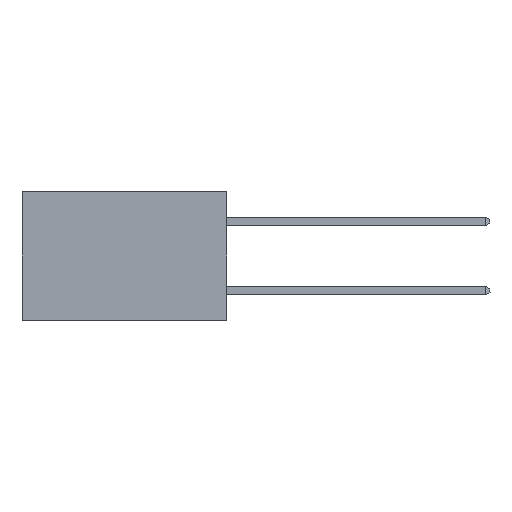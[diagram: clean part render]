
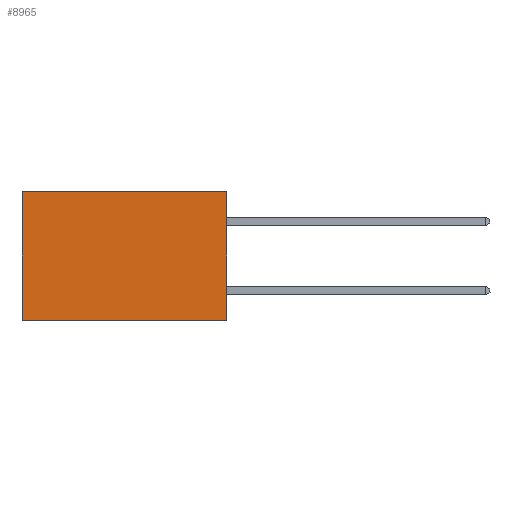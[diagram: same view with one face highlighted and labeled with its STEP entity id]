
A CAD part, left-side view. The second image highlights one B-rep face of the part: STEP entity #8965.
In plain terms, the highlighted planar face has unit normal (-1, 0, 0).
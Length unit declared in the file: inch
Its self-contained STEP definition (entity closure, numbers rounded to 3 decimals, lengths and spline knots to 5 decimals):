
#367 = CARTESIAN_POINT ( 'NONE',  ( 0.277, 0., 0. ) ) ;
#371 = VERTEX_POINT ( 'NONE', #10966 ) ;
#511 = VECTOR ( 'NONE', #11089, 39.37008 ) ;
#581 = VECTOR ( 'NONE', #9705, 39.37008 ) ;
#585 = ORIENTED_EDGE ( 'NONE', *, *, #1440, .F. ) ;
#1276 = AXIS2_PLACEMENT_3D ( 'NONE', #5272, #8600, #3576 ) ;
#1440 = EDGE_CURVE ( 'NONE', #1520, #371, #10931, .T. ) ;
#1470 = VERTEX_POINT ( 'NONE', #6019 ) ;
#1520 = VERTEX_POINT ( 'NONE', #367 ) ;
#1776 = CARTESIAN_POINT ( 'NONE',  ( 0.277, 0.59, 0. ) ) ;
#2143 = VECTOR ( 'NONE', #6557, 39.37008 ) ;
#2701 = PLANE ( 'NONE',  #1276 ) ;
#2842 = ORIENTED_EDGE ( 'NONE', *, *, #4392, .T. ) ;
#3112 = LINE ( 'NONE', #10121, #581 ) ;
#3576 = DIRECTION ( 'NONE',  ( 0., 0., -1. ) ) ;
#3627 = CARTESIAN_POINT ( 'NONE',  ( 0.277, 0., -0.37 ) ) ;
#3794 = EDGE_CURVE ( 'NONE', #371, #1470, #6707, .T. ) ;
#3947 = VERTEX_POINT ( 'NONE', #1776 ) ;
#4392 = EDGE_CURVE ( 'NONE', #3947, #1470, #3112, .T. ) ;
#4713 = FACE_OUTER_BOUND ( 'NONE', #7220, .T. ) ;
#5272 = CARTESIAN_POINT ( 'NONE',  ( 0.277, 0., -0.37 ) ) ;
#5414 = ORIENTED_EDGE ( 'NONE', *, *, #9619, .T. ) ;
#6019 = CARTESIAN_POINT ( 'NONE',  ( 0.277, 0.59, -0.37 ) ) ;
#6138 = CARTESIAN_POINT ( 'NONE',  ( 0.277, 0., 0. ) ) ;
#6557 = DIRECTION ( 'NONE',  ( 0., 1., 0. ) ) ;
#6707 = LINE ( 'NONE', #3627, #2143 ) ;
#7220 = EDGE_LOOP ( 'NONE', ( #2842, #9615, #585, #5414 ) ) ;
#8600 = DIRECTION ( 'NONE',  ( 1., 0., 0. ) ) ;
#8965 = ADVANCED_FACE ( 'NONE', ( #4713 ), #2701, .F. ) ;
#9615 = ORIENTED_EDGE ( 'NONE', *, *, #3794, .F. ) ;
#9619 = EDGE_CURVE ( 'NONE', #1520, #3947, #10086, .T. ) ;
#9705 = DIRECTION ( 'NONE',  ( 0., 0., -1. ) ) ;
#10086 = LINE ( 'NONE', #6138, #511 ) ;
#10121 = CARTESIAN_POINT ( 'NONE',  ( 0.277, 0.59, -0.37 ) ) ;
#10321 = DIRECTION ( 'NONE',  ( 0., 0., -1. ) ) ;
#10838 = CARTESIAN_POINT ( 'NONE',  ( 0.277, 0., -0.37 ) ) ;
#10931 = LINE ( 'NONE', #10838, #11177 ) ;
#10966 = CARTESIAN_POINT ( 'NONE',  ( 0.277, 0., -0.37 ) ) ;
#11089 = DIRECTION ( 'NONE',  ( 0., 1., 0. ) ) ;
#11177 = VECTOR ( 'NONE', #10321, 39.37008 ) ;
